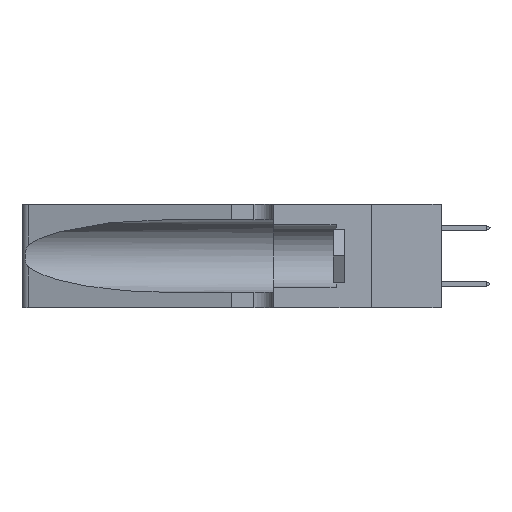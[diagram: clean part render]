
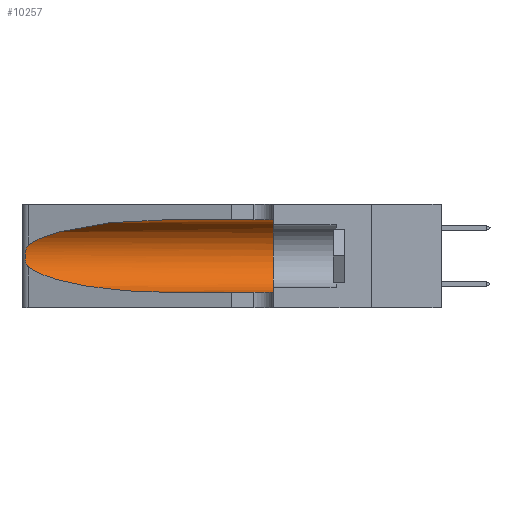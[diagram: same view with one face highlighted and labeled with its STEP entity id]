
A CAD part, left-side view. The second image highlights one B-rep face of the part: STEP entity #10257.
In plain terms, the highlighted cylindrical face has radius 3.308 mm (diameter 6.617 mm), a partial arc.
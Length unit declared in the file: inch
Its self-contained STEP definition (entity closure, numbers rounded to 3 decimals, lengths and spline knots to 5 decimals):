
#2162 = CARTESIAN_POINT ( 'NONE',  ( 0.26017, 1.23833, 0.17102 ) ) ;
#2280 = CARTESIAN_POINT ( 'NONE',  ( 0.1305, 0.35, 0.05475 ) ) ;
#3507 = LINE ( 'NONE', #25300, #35905 ) ;
#5125 = CARTESIAN_POINT ( 'NONE',  ( 0.18966, 0.96281, 0.31525 ) ) ;
#5624 = DIRECTION ( 'NONE',  ( 0., 0., -1. ) ) ;
#5776 = CARTESIAN_POINT ( 'NONE',  ( 0.25854, 1.2359, 0.20912 ) ) ;
#6515 = CARTESIAN_POINT ( 'NONE',  ( 0.25487, 1.22718, 0.22369 ) ) ;
#6733 = VECTOR ( 'NONE', #35050, 39.37008 ) ;
#8291 = EDGE_LOOP ( 'NONE', ( #26151, #24781, #29148, #11818, #13313, #9212 ) ) ;
#9212 = ORIENTED_EDGE ( 'NONE', *, *, #19294, .F. ) ;
#10257 = ADVANCED_FACE ( 'NONE', ( #16888 ), #13347, .F. ) ;
#11425 = DIRECTION ( 'NONE',  ( 0., 1., 0. ) ) ;
#11506 = CARTESIAN_POINT ( 'NONE',  ( 0.1305, 1.61858, 0.05475 ) ) ;
#11818 = ORIENTED_EDGE ( 'NONE', *, *, #29324, .T. ) ;
#12187 = CARTESIAN_POINT ( 'NONE',  ( 0.25856, 1.23593, 0.16098 ) ) ;
#13313 = ORIENTED_EDGE ( 'NONE', *, *, #28425, .F. ) ;
#13347 = CYLINDRICAL_SURFACE ( 'NONE', #28140, 0.13025 ) ;
#13468 = CIRCLE ( 'NONE', #17211, 0.13025 ) ;
#15374 = CARTESIAN_POINT ( 'NONE',  ( 0.26075, 1.23896, 0.19203 ) ) ;
#15641 = CARTESIAN_POINT ( 'NONE',  ( 0.25639, 1.23186, 0.15144 ) ) ;
#16888 = FACE_OUTER_BOUND ( 'NONE', #8291, .T. ) ;
#17085 =( BOUNDED_CURVE ( )  B_SPLINE_CURVE ( 3, ( #24945, #31386, #25229, #28526 ),
 .UNSPECIFIED., .F., .T. ) 
 B_SPLINE_CURVE_WITH_KNOTS ( ( 4, 4 ),
 ( 3.44316, 4.71239 ),
 .UNSPECIFIED. ) 
 CURVE ( )  GEOMETRIC_REPRESENTATION_ITEM ( )  RATIONAL_B_SPLINE_CURVE ( ( 1., 0.87, 0.87, 1. ) ) 
 REPRESENTATION_ITEM ( '' )  );
#17211 = AXIS2_PLACEMENT_3D ( 'NONE', #27783, #11425, #31227 ) ;
#17415 = VERTEX_POINT ( 'NONE', #2280 ) ;
#18069 = CARTESIAN_POINT ( 'NONE',  ( 0.25487, 1.22718, 0.22369 ) ) ;
#18513 = CARTESIAN_POINT ( 'NONE',  ( 0.25787, 1.23484, 0.2124 ) ) ;
#19294 = EDGE_CURVE ( 'NONE', #26103, #38209, #3507, .T. ) ;
#19353 = VERTEX_POINT ( 'NONE', #37966 ) ;
#20536 = DIRECTION ( 'NONE',  ( 0., -1., 0. ) ) ;
#21357 = CARTESIAN_POINT ( 'NONE',  ( 0.25555, 1.22994, 0.2215 ) ) ;
#24781 = ORIENTED_EDGE ( 'NONE', *, *, #27890, .T. ) ;
#24800 =( BOUNDED_CURVE ( )  B_SPLINE_CURVE ( 3, ( #28638, #5125, #31492, #37952 ),
 .UNSPECIFIED., .F., .F. ) 
 B_SPLINE_CURVE_WITH_KNOTS ( ( 4, 4 ),
 ( 1.5708, 2.84003 ),
 .UNSPECIFIED. ) 
 CURVE ( )  GEOMETRIC_REPRESENTATION_ITEM ( )  RATIONAL_B_SPLINE_CURVE ( ( 1., 0.87, 0.87, 1. ) ) 
 REPRESENTATION_ITEM ( '' )  );
#24945 = CARTESIAN_POINT ( 'NONE',  ( 0.25487, 1.22718, 0.14631 ) ) ;
#25229 = CARTESIAN_POINT ( 'NONE',  ( 0.18966, 0.96281, 0.05475 ) ) ;
#25300 = CARTESIAN_POINT ( 'NONE',  ( 0.1305, 1.61858, 0.31525 ) ) ;
#26103 = VERTEX_POINT ( 'NONE', #34010 ) ;
#26151 = ORIENTED_EDGE ( 'NONE', *, *, #36319, .T. ) ;
#27783 = CARTESIAN_POINT ( 'NONE',  ( 0.1305, 0.35, 0.185 ) ) ;
#27890 = EDGE_CURVE ( 'NONE', #36351, #36132, #30522, .T. ) ;
#28140 = AXIS2_PLACEMENT_3D ( 'NONE', #31400, #35000, #5624 ) ;
#28425 = EDGE_CURVE ( 'NONE', #38209, #17415, #13468, .T. ) ;
#28473 = CARTESIAN_POINT ( 'NONE',  ( 0.1305, 0.35, 0.31525 ) ) ;
#28503 = CARTESIAN_POINT ( 'NONE',  ( 0.25487, 1.22718, 0.14631 ) ) ;
#28526 = CARTESIAN_POINT ( 'NONE',  ( 0.1305, 0.72297, 0.05475 ) ) ;
#28638 = CARTESIAN_POINT ( 'NONE',  ( 0.1305, 0.72297, 0.31525 ) ) ;
#28696 = CARTESIAN_POINT ( 'NONE',  ( 0.25789, 1.23486, 0.15765 ) ) ;
#29148 = ORIENTED_EDGE ( 'NONE', *, *, #40587, .T. ) ;
#29324 = EDGE_CURVE ( 'NONE', #19353, #17415, #42135, .T. ) ;
#30522 = B_SPLINE_CURVE_WITH_KNOTS ( 'NONE', 3,
 ( #18069, #21357, #37866, #18513, #5776, #41864, #15374, #31843, #2162, #12187, #28696, #15641, #41721, #38569 ),
 .UNSPECIFIED., .F., .F.,
 ( 4, 2, 2, 2, 2, 2, 4 ),
 ( 0., 0.00027, 0.00053, 0.00107, 0.0016, 0.00187, 0.00214 ),
 .UNSPECIFIED. ) ;
#31227 = DIRECTION ( 'NONE',  ( 0., 0., 1. ) ) ;
#31386 = CARTESIAN_POINT ( 'NONE',  ( 0.2373, 1.15595, 0.08982 ) ) ;
#31400 = CARTESIAN_POINT ( 'NONE',  ( 0.1305, 1.61858, 0.185 ) ) ;
#31492 = CARTESIAN_POINT ( 'NONE',  ( 0.2373, 1.15595, 0.28018 ) ) ;
#31843 = CARTESIAN_POINT ( 'NONE',  ( 0.26075, 1.23896, 0.178 ) ) ;
#34010 = CARTESIAN_POINT ( 'NONE',  ( 0.1305, 0.72297, 0.31525 ) ) ;
#35000 = DIRECTION ( 'NONE',  ( 0., -1., 0. ) ) ;
#35050 = DIRECTION ( 'NONE',  ( 0., -1., 0. ) ) ;
#35905 = VECTOR ( 'NONE', #20536, 39.37008 ) ;
#36132 = VERTEX_POINT ( 'NONE', #28503 ) ;
#36319 = EDGE_CURVE ( 'NONE', #26103, #36351, #24800, .T. ) ;
#36351 = VERTEX_POINT ( 'NONE', #6515 ) ;
#37866 = CARTESIAN_POINT ( 'NONE',  ( 0.25639, 1.23184, 0.21858 ) ) ;
#37952 = CARTESIAN_POINT ( 'NONE',  ( 0.25487, 1.22718, 0.22369 ) ) ;
#37966 = CARTESIAN_POINT ( 'NONE',  ( 0.1305, 0.72297, 0.05475 ) ) ;
#38209 = VERTEX_POINT ( 'NONE', #28473 ) ;
#38569 = CARTESIAN_POINT ( 'NONE',  ( 0.25487, 1.22718, 0.14631 ) ) ;
#40587 = EDGE_CURVE ( 'NONE', #36132, #19353, #17085, .T. ) ;
#41721 = CARTESIAN_POINT ( 'NONE',  ( 0.25555, 1.22993, 0.14849 ) ) ;
#41864 = CARTESIAN_POINT ( 'NONE',  ( 0.26018, 1.23835, 0.19895 ) ) ;
#42135 = LINE ( 'NONE', #11506, #6733 ) ;
